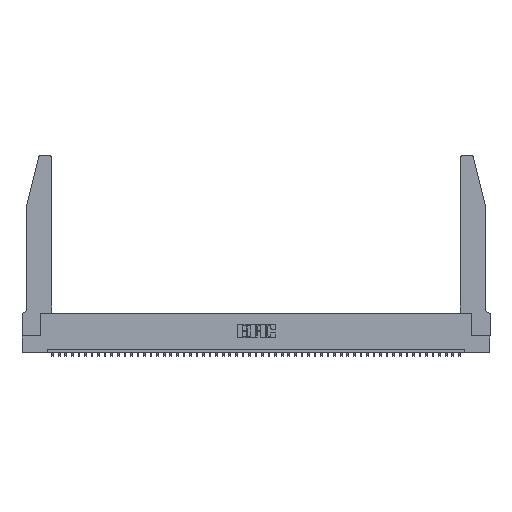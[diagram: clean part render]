
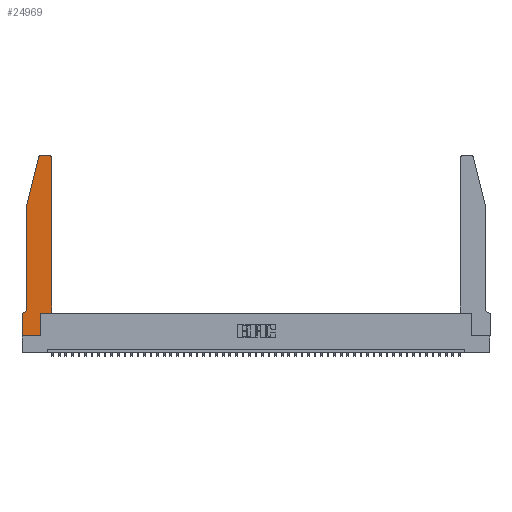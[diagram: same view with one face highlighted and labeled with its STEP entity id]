
A CAD part, top view. The second image highlights one B-rep face of the part: STEP entity #24969.
In plain terms, the highlighted planar face has unit normal (0, 0, 1).
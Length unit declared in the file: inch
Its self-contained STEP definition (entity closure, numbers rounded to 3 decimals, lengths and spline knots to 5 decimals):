
#281 = CARTESIAN_POINT ( 'NONE',  ( 0.0055, 0.35, 0.37 ) ) ;
#444 = CIRCLE ( 'NONE', #28223, 0.03 ) ;
#758 = DIRECTION ( 'NONE',  ( 0., 1., 0. ) ) ;
#2319 = ORIENTED_EDGE ( 'NONE', *, *, #35619, .T. ) ;
#2664 = CARTESIAN_POINT ( 'NONE',  ( 0.284, 2.72, 0.37 ) ) ;
#3272 = PLANE ( 'NONE',  #33758 ) ;
#5481 = CARTESIAN_POINT ( 'NONE',  ( 0.4205, 2.75, 0.37 ) ) ;
#5868 = EDGE_CURVE ( 'NONE', #32206, #39409, #22126, .T. ) ;
#6292 = ORIENTED_EDGE ( 'NONE', *, *, #31264, .T. ) ;
#6506 = VECTOR ( 'NONE', #758, 39.37008 ) ;
#6638 = DIRECTION ( 'NONE',  ( -0.239, -0.971, 0. ) ) ;
#7035 = DIRECTION ( 'NONE',  ( 0., 0., 1. ) ) ;
#7304 = EDGE_CURVE ( 'NONE', #8057, #25934, #38624, .T. ) ;
#8057 = VERTEX_POINT ( 'NONE', #10774 ) ;
#8744 = CARTESIAN_POINT ( 'NONE',  ( 0.2865, 0.35, 0.37 ) ) ;
#9506 = CARTESIAN_POINT ( 'NONE',  ( 0.4505, 0.35, 0.37 ) ) ;
#9520 = EDGE_CURVE ( 'NONE', #25934, #38917, #34263, .T. ) ;
#10206 = LINE ( 'NONE', #16345, #41740 ) ;
#10336 = CARTESIAN_POINT ( 'NONE',  ( 0.2605, 2.75, 0.37 ) ) ;
#10624 = ORIENTED_EDGE ( 'NONE', *, *, #33034, .T. ) ;
#10774 = CARTESIAN_POINT ( 'NONE',  ( 0.2865, 0., 0.37 ) ) ;
#11507 = DIRECTION ( 'NONE',  ( 1., 0., 0. ) ) ;
#12211 = CARTESIAN_POINT ( 'NONE',  ( 0.4505, 2.72, 0.37 ) ) ;
#13119 = LINE ( 'NONE', #20326, #36839 ) ;
#14284 = CARTESIAN_POINT ( 'NONE',  ( 0.4505, 0.35, 0.37 ) ) ;
#15378 = EDGE_CURVE ( 'NONE', #41248, #46606, #35961, .T. ) ;
#15469 = ORIENTED_EDGE ( 'NONE', *, *, #15378, .T. ) ;
#15996 = ORIENTED_EDGE ( 'NONE', *, *, #9520, .T. ) ;
#16007 = EDGE_LOOP ( 'NONE', ( #24880, #46419, #15469, #6292, #10624, #24869, #44844, #36776, #40191, #15996, #30345, #2319 ) ) ;
#16157 = CARTESIAN_POINT ( 'NONE',  ( 0.0055, 0.42, 0.37 ) ) ;
#16345 = CARTESIAN_POINT ( 'NONE',  ( 0., 0., 0.37 ) ) ;
#16427 = VECTOR ( 'NONE', #31770, 39.37008 ) ;
#16708 = DIRECTION ( 'NONE',  ( -1., 0., 0. ) ) ;
#16893 = CIRCLE ( 'NONE', #27200, 0.07 ) ;
#18308 = CARTESIAN_POINT ( 'NONE',  ( 0.0755, 2., 0.37 ) ) ;
#18526 = FACE_OUTER_BOUND ( 'NONE', #16007, .T. ) ;
#19242 = VECTOR ( 'NONE', #44674, 39.37008 ) ;
#19449 = DIRECTION ( 'NONE',  ( 0., 0., 1. ) ) ;
#20230 = CARTESIAN_POINT ( 'NONE',  ( 0., 0., 0.37 ) ) ;
#20278 = LINE ( 'NONE', #23812, #23214 ) ;
#20326 = CARTESIAN_POINT ( 'NONE',  ( 0.0755, 0.35, 0.37 ) ) ;
#21010 = LINE ( 'NONE', #14284, #19242 ) ;
#21953 = CARTESIAN_POINT ( 'NONE',  ( 0., 0.35, 0.37 ) ) ;
#22126 = LINE ( 'NONE', #10336, #30417 ) ;
#22200 = CARTESIAN_POINT ( 'NONE',  ( 0.2865, 0.35, 0.37 ) ) ;
#23214 = VECTOR ( 'NONE', #27650, 39.37008 ) ;
#23812 = CARTESIAN_POINT ( 'NONE',  ( 0., 0., 0.37 ) ) ;
#24182 = CARTESIAN_POINT ( 'NONE',  ( 0.0755, 0.42, 0.37 ) ) ;
#24869 = ORIENTED_EDGE ( 'NONE', *, *, #25612, .T. ) ;
#24880 = ORIENTED_EDGE ( 'NONE', *, *, #5868, .T. ) ;
#24969 = ADVANCED_FACE ( 'NONE', ( #18526 ), #3272, .T. ) ;
#25612 = EDGE_CURVE ( 'NONE', #48420, #48430, #13119, .T. ) ;
#25934 = VERTEX_POINT ( 'NONE', #22200 ) ;
#27200 = AXIS2_PLACEMENT_3D ( 'NONE', #16157, #27392, #39027 ) ;
#27392 = DIRECTION ( 'NONE',  ( 0., 0., -1. ) ) ;
#27650 = DIRECTION ( 'NONE',  ( 1., 0., 0. ) ) ;
#28136 = CARTESIAN_POINT ( 'NONE',  ( 0.284, 2.75, 0.37 ) ) ;
#28223 = AXIS2_PLACEMENT_3D ( 'NONE', #29325, #7035, #41309 ) ;
#29325 = CARTESIAN_POINT ( 'NONE',  ( 0.4205, 2.72, 0.37 ) ) ;
#30345 = ORIENTED_EDGE ( 'NONE', *, *, #46169, .T. ) ;
#30369 = CARTESIAN_POINT ( 'NONE',  ( 0., 0.35, 0.37 ) ) ;
#30417 = VECTOR ( 'NONE', #44752, 39.37008 ) ;
#30559 = EDGE_CURVE ( 'NONE', #47155, #8057, #20278, .T. ) ;
#30721 = VERTEX_POINT ( 'NONE', #12211 ) ;
#31264 = EDGE_CURVE ( 'NONE', #46606, #48027, #41659, .T. ) ;
#31770 = DIRECTION ( 'NONE',  ( 1., 0., 0. ) ) ;
#32206 = VERTEX_POINT ( 'NONE', #5481 ) ;
#33034 = EDGE_CURVE ( 'NONE', #48027, #48420, #16893, .T. ) ;
#33345 = CARTESIAN_POINT ( 'NONE',  ( 0.4505, 0.35, 0.37 ) ) ;
#33758 = AXIS2_PLACEMENT_3D ( 'NONE', #21953, #19449, #11507 ) ;
#34263 = LINE ( 'NONE', #33345, #16427 ) ;
#35619 = EDGE_CURVE ( 'NONE', #30721, #32206, #444, .T. ) ;
#35961 = LINE ( 'NONE', #47958, #38873 ) ;
#36707 = EDGE_CURVE ( 'NONE', #39409, #41248, #42679, .T. ) ;
#36776 = ORIENTED_EDGE ( 'NONE', *, *, #30559, .T. ) ;
#36839 = VECTOR ( 'NONE', #16708, 39.37008 ) ;
#38624 = LINE ( 'NONE', #8744, #6506 ) ;
#38764 = EDGE_CURVE ( 'NONE', #48430, #47155, #10206, .T. ) ;
#38873 = VECTOR ( 'NONE', #6638, 39.37008 ) ;
#38917 = VERTEX_POINT ( 'NONE', #9506 ) ;
#39027 = DIRECTION ( 'NONE',  ( -1., 0., 0. ) ) ;
#39377 = CARTESIAN_POINT ( 'NONE',  ( 0.0755, 2., 0.37 ) ) ;
#39409 = VERTEX_POINT ( 'NONE', #28136 ) ;
#40191 = ORIENTED_EDGE ( 'NONE', *, *, #7304, .T. ) ;
#41248 = VERTEX_POINT ( 'NONE', #43316 ) ;
#41309 = DIRECTION ( 'NONE',  ( 1., 0., 0. ) ) ;
#41315 = DIRECTION ( 'NONE',  ( 0., 0., 1. ) ) ;
#41659 = LINE ( 'NONE', #18308, #49436 ) ;
#41740 = VECTOR ( 'NONE', #43588, 39.37008 ) ;
#42679 = CIRCLE ( 'NONE', #49392, 0.03 ) ;
#43316 = CARTESIAN_POINT ( 'NONE',  ( 0.25487, 2.72718, 0.37 ) ) ;
#43588 = DIRECTION ( 'NONE',  ( 0., -1., 0. ) ) ;
#44568 = DIRECTION ( 'NONE',  ( 0., -1., 0. ) ) ;
#44674 = DIRECTION ( 'NONE',  ( 0., 1., 0. ) ) ;
#44752 = DIRECTION ( 'NONE',  ( -1., 0., 0. ) ) ;
#44844 = ORIENTED_EDGE ( 'NONE', *, *, #38764, .T. ) ;
#46169 = EDGE_CURVE ( 'NONE', #38917, #30721, #21010, .T. ) ;
#46419 = ORIENTED_EDGE ( 'NONE', *, *, #36707, .T. ) ;
#46606 = VERTEX_POINT ( 'NONE', #39377 ) ;
#47155 = VERTEX_POINT ( 'NONE', #20230 ) ;
#47958 = CARTESIAN_POINT ( 'NONE',  ( 0.0755, 2., 0.37 ) ) ;
#48027 = VERTEX_POINT ( 'NONE', #24182 ) ;
#48420 = VERTEX_POINT ( 'NONE', #281 ) ;
#48430 = VERTEX_POINT ( 'NONE', #30369 ) ;
#48532 = DIRECTION ( 'NONE',  ( 1., 0., 0. ) ) ;
#49392 = AXIS2_PLACEMENT_3D ( 'NONE', #2664, #41315, #48532 ) ;
#49436 = VECTOR ( 'NONE', #44568, 39.37008 ) ;
